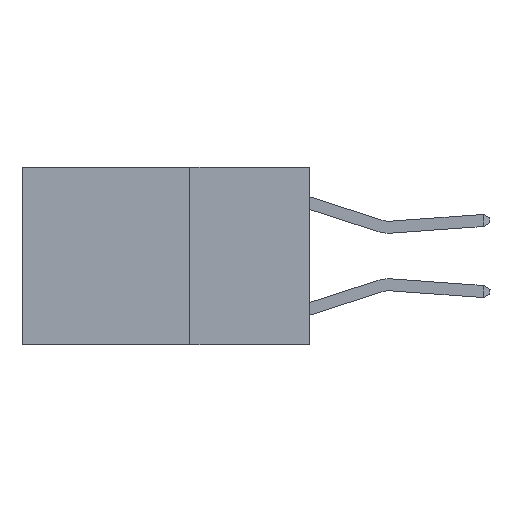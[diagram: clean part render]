
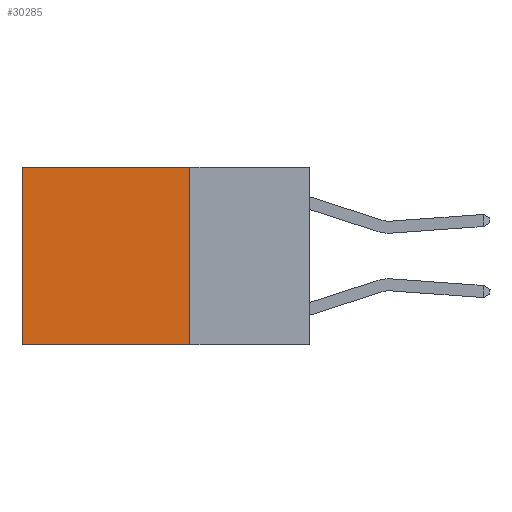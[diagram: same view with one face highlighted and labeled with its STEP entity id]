
A CAD part, left-side view. The second image highlights one B-rep face of the part: STEP entity #30285.
In plain terms, the highlighted planar face has unit normal (-1, 0, 0).
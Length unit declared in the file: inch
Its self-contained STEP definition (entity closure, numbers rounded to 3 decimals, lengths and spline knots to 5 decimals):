
#63 = DIRECTION ( 'NONE',  ( 0., 0., -1. ) ) ;
#589 = CARTESIAN_POINT ( 'NONE',  ( 0.2625, 0.25, 0. ) ) ;
#759 = EDGE_CURVE ( 'NONE', #16078, #25974, #12110, .T. ) ;
#3367 = CARTESIAN_POINT ( 'NONE',  ( 0.2625, 0.25, 0. ) ) ;
#3603 = CARTESIAN_POINT ( 'NONE',  ( 0.2625, 0.6, -0.37 ) ) ;
#5077 = EDGE_CURVE ( 'NONE', #19468, #25974, #11800, .T. ) ;
#6198 = VECTOR ( 'NONE', #63, 39.37008 ) ;
#7097 = DIRECTION ( 'NONE',  ( 0., 1., 0. ) ) ;
#9928 = LINE ( 'NONE', #17080, #28290 ) ;
#10105 = LINE ( 'NONE', #589, #28465 ) ;
#10284 = EDGE_CURVE ( 'NONE', #16724, #16078, #9928, .T. ) ;
#10629 = DIRECTION ( 'NONE',  ( 0., 0., -1. ) ) ;
#11800 = LINE ( 'NONE', #31823, #30142 ) ;
#12110 = LINE ( 'NONE', #22490, #6198 ) ;
#12260 = EDGE_LOOP ( 'NONE', ( #22496, #24229, #28779, #13701 ) ) ;
#13701 = ORIENTED_EDGE ( 'NONE', *, *, #10284, .T. ) ;
#16078 = VERTEX_POINT ( 'NONE', #18515 ) ;
#16335 = FACE_OUTER_BOUND ( 'NONE', #12260, .T. ) ;
#16724 = VERTEX_POINT ( 'NONE', #3367 ) ;
#17080 = CARTESIAN_POINT ( 'NONE',  ( 0.2625, 0.25, 0. ) ) ;
#18515 = CARTESIAN_POINT ( 'NONE',  ( 0.2625, 0.6, 0. ) ) ;
#19468 = VERTEX_POINT ( 'NONE', #23265 ) ;
#20565 = PLANE ( 'NONE',  #26346 ) ;
#22490 = CARTESIAN_POINT ( 'NONE',  ( 0.2625, 0.6, 0. ) ) ;
#22496 = ORIENTED_EDGE ( 'NONE', *, *, #759, .T. ) ;
#23265 = CARTESIAN_POINT ( 'NONE',  ( 0.2625, 0.25, -0.37 ) ) ;
#24229 = ORIENTED_EDGE ( 'NONE', *, *, #5077, .F. ) ;
#25603 = DIRECTION ( 'NONE',  ( 1., 0., 0. ) ) ;
#25974 = VERTEX_POINT ( 'NONE', #3603 ) ;
#26346 = AXIS2_PLACEMENT_3D ( 'NONE', #30494, #25603, #10629 ) ;
#27736 = EDGE_CURVE ( 'NONE', #16724, #19468, #10105, .T. ) ;
#28290 = VECTOR ( 'NONE', #7097, 39.37008 ) ;
#28465 = VECTOR ( 'NONE', #30629, 39.37008 ) ;
#28779 = ORIENTED_EDGE ( 'NONE', *, *, #27736, .F. ) ;
#29441 = DIRECTION ( 'NONE',  ( 0., 1., 0. ) ) ;
#30142 = VECTOR ( 'NONE', #29441, 39.37008 ) ;
#30285 = ADVANCED_FACE ( 'NONE', ( #16335 ), #20565, .F. ) ;
#30494 = CARTESIAN_POINT ( 'NONE',  ( 0.2625, 0.25, 0. ) ) ;
#30629 = DIRECTION ( 'NONE',  ( 0., 0., -1. ) ) ;
#31823 = CARTESIAN_POINT ( 'NONE',  ( 0.2625, 0.25, -0.37 ) ) ;
